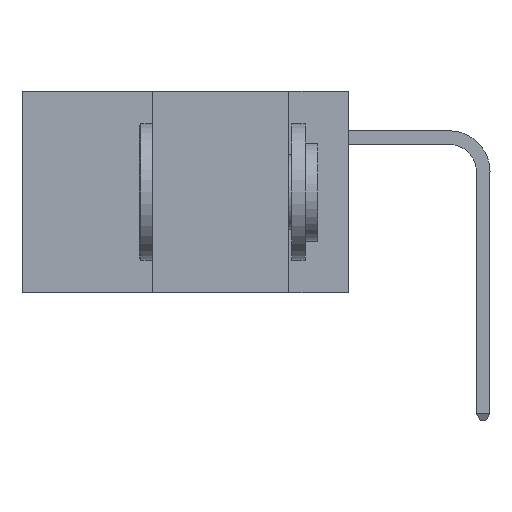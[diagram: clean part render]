
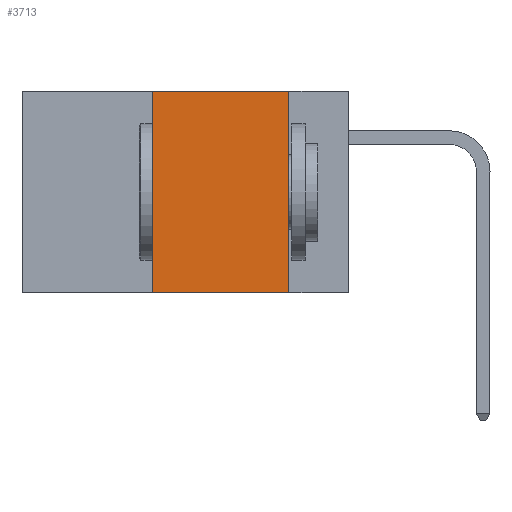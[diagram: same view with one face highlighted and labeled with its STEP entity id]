
A CAD part, left-side view. The second image highlights one B-rep face of the part: STEP entity #3713.
In plain terms, the highlighted planar face has unit normal (-1, 0, 0).
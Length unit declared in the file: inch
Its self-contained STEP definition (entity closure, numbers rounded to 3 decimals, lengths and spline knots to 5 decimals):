
#1880 = VECTOR ( 'NONE', #11407, 39.37008 ) ;
#1990 = ORIENTED_EDGE ( 'NONE', *, *, #7714, .F. ) ;
#2923 = CARTESIAN_POINT ( 'NONE',  ( 0., 0.6, -0.37 ) ) ;
#3225 = CARTESIAN_POINT ( 'NONE',  ( 0., 0.36, 0. ) ) ;
#3713 = ADVANCED_FACE ( 'NONE', ( #19480 ), #5772, .F. ) ;
#4470 = VECTOR ( 'NONE', #5953, 39.37008 ) ;
#4486 = AXIS2_PLACEMENT_3D ( 'NONE', #5864, #9994, #24592 ) ;
#4564 = VECTOR ( 'NONE', #12486, 39.37008 ) ;
#4970 = ORIENTED_EDGE ( 'NONE', *, *, #9405, .F. ) ;
#5772 = PLANE ( 'NONE',  #4486 ) ;
#5864 = CARTESIAN_POINT ( 'NONE',  ( 0., 0.6, 0. ) ) ;
#5953 = DIRECTION ( 'NONE',  ( 0., -1., 0. ) ) ;
#7714 = EDGE_CURVE ( 'NONE', #9840, #25789, #10030, .T. ) ;
#9111 = EDGE_CURVE ( 'NONE', #23789, #25789, #12922, .T. ) ;
#9405 = EDGE_CURVE ( 'NONE', #22830, #9840, #10587, .T. ) ;
#9840 = VERTEX_POINT ( 'NONE', #23133 ) ;
#9934 = CARTESIAN_POINT ( 'NONE',  ( 0., 0.11, -0.37 ) ) ;
#9994 = DIRECTION ( 'NONE',  ( 1., 0., 0. ) ) ;
#10030 = LINE ( 'NONE', #18814, #4564 ) ;
#10587 = LINE ( 'NONE', #24596, #4470 ) ;
#11407 = DIRECTION ( 'NONE',  ( 0., 0., 1. ) ) ;
#12368 = ORIENTED_EDGE ( 'NONE', *, *, #23129, .F. ) ;
#12486 = DIRECTION ( 'NONE',  ( 0., 0., -1. ) ) ;
#12922 = LINE ( 'NONE', #2923, #17823 ) ;
#13606 = CARTESIAN_POINT ( 'NONE',  ( 0., 0.36, -0.37 ) ) ;
#13713 = ORIENTED_EDGE ( 'NONE', *, *, #9111, .T. ) ;
#16678 = CARTESIAN_POINT ( 'NONE',  ( 0., 0.36, 0. ) ) ;
#17823 = VECTOR ( 'NONE', #21666, 39.37008 ) ;
#18498 = LINE ( 'NONE', #3225, #1880 ) ;
#18814 = CARTESIAN_POINT ( 'NONE',  ( 0., 0.11, 0. ) ) ;
#19480 = FACE_OUTER_BOUND ( 'NONE', #21546, .T. ) ;
#21546 = EDGE_LOOP ( 'NONE', ( #1990, #4970, #12368, #13713 ) ) ;
#21666 = DIRECTION ( 'NONE',  ( 0., -1., 0. ) ) ;
#22830 = VERTEX_POINT ( 'NONE', #16678 ) ;
#23129 = EDGE_CURVE ( 'NONE', #23789, #22830, #18498, .T. ) ;
#23133 = CARTESIAN_POINT ( 'NONE',  ( 0., 0.11, 0. ) ) ;
#23789 = VERTEX_POINT ( 'NONE', #13606 ) ;
#24592 = DIRECTION ( 'NONE',  ( 0., 0., -1. ) ) ;
#24596 = CARTESIAN_POINT ( 'NONE',  ( 0., 0.6, 0. ) ) ;
#25789 = VERTEX_POINT ( 'NONE', #9934 ) ;
